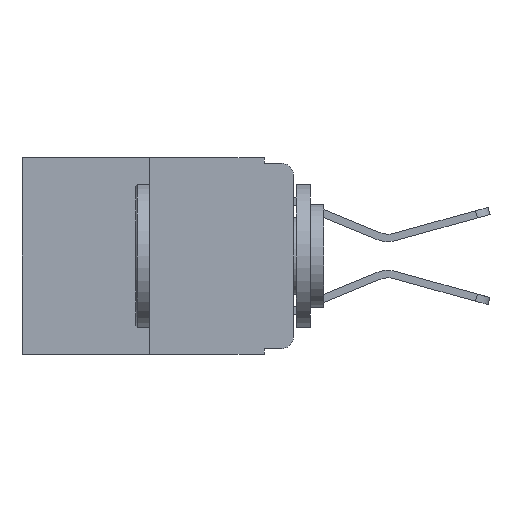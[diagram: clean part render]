
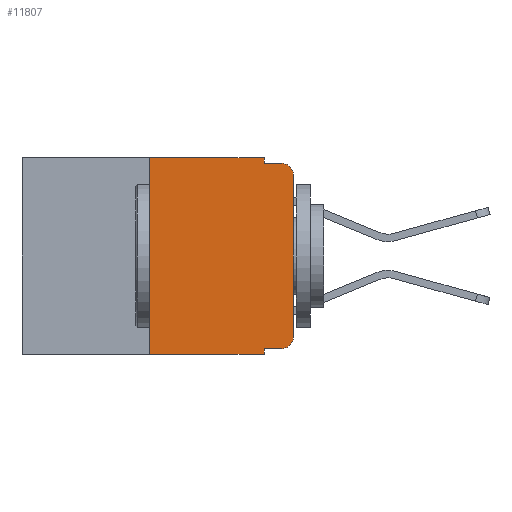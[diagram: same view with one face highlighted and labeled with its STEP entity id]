
A CAD part, left-side view. The second image highlights one B-rep face of the part: STEP entity #11807.
In plain terms, the highlighted planar face has unit normal (-1, 0, 0).
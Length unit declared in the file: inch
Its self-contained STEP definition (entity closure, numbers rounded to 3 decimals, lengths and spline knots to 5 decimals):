
#235 = ORIENTED_EDGE ( 'NONE', *, *, #6135, .F. ) ;
#460 = ORIENTED_EDGE ( 'NONE', *, *, #6069, .F. ) ;
#597 = LINE ( 'NONE', #14722, #12725 ) ;
#1324 = LINE ( 'NONE', #8059, #4423 ) ;
#1347 = DIRECTION ( 'NONE',  ( 0., 0., -1. ) ) ;
#1419 = VERTEX_POINT ( 'NONE', #8346 ) ;
#1439 = CARTESIAN_POINT ( 'NONE',  ( 0., 0.473, -0.343 ) ) ;
#1730 = LINE ( 'NONE', #14978, #10728 ) ;
#2251 = CARTESIAN_POINT ( 'NONE',  ( 0., 0.25, -0.343 ) ) ;
#2420 = CARTESIAN_POINT ( 'NONE',  ( 0., 0.051, -0.343 ) ) ;
#2587 = CARTESIAN_POINT ( 'NONE',  ( 0., 0.051, -0.01 ) ) ;
#2831 = DIRECTION ( 'NONE',  ( 0., -1., 0. ) ) ;
#3692 = ORIENTED_EDGE ( 'NONE', *, *, #5972, .T. ) ;
#3887 = ORIENTED_EDGE ( 'NONE', *, *, #6138, .T. ) ;
#3972 = CARTESIAN_POINT ( 'NONE',  ( 0., 0.25, 0. ) ) ;
#3984 = VECTOR ( 'NONE', #1347, 39.37008 ) ;
#4053 = VERTEX_POINT ( 'NONE', #5245 ) ;
#4377 = LINE ( 'NONE', #11861, #3984 ) ;
#4423 = VECTOR ( 'NONE', #5889, 39.37008 ) ;
#4670 = VERTEX_POINT ( 'NONE', #5679 ) ;
#5110 = DIRECTION ( 'NONE',  ( -1., 0., 0. ) ) ;
#5166 = EDGE_CURVE ( 'NONE', #1419, #8524, #1324, .T. ) ;
#5201 = PLANE ( 'NONE',  #5673 ) ;
#5245 = CARTESIAN_POINT ( 'NONE',  ( 0., 0.02, -0.333 ) ) ;
#5320 = CARTESIAN_POINT ( 'NONE',  ( 0., 0.051, -0.333 ) ) ;
#5601 = DIRECTION ( 'NONE',  ( -1., 0., 0. ) ) ;
#5673 = AXIS2_PLACEMENT_3D ( 'NONE', #13996, #7548, #15067 ) ;
#5679 = CARTESIAN_POINT ( 'NONE',  ( 0., 0.051, -0.333 ) ) ;
#5693 = EDGE_CURVE ( 'NONE', #7178, #12942, #8194, .T. ) ;
#5730 = CARTESIAN_POINT ( 'NONE',  ( 0., 0., -0.313 ) ) ;
#5889 = DIRECTION ( 'NONE',  ( 0., -1., 0. ) ) ;
#5972 = EDGE_CURVE ( 'NONE', #9551, #14573, #597, .T. ) ;
#6068 = EDGE_CURVE ( 'NONE', #14573, #13888, #11398, .T. ) ;
#6069 = EDGE_CURVE ( 'NONE', #8213, #13888, #13911, .T. ) ;
#6073 = CARTESIAN_POINT ( 'NONE',  ( 0., 0., -0.03 ) ) ;
#6095 = EDGE_CURVE ( 'NONE', #8524, #8213, #1730, .T. ) ;
#6115 = EDGE_CURVE ( 'NONE', #7178, #1419, #13583, .T. ) ;
#6135 = EDGE_CURVE ( 'NONE', #4670, #12942, #4377, .T. ) ;
#6138 = EDGE_CURVE ( 'NONE', #4670, #4053, #9695, .T. ) ;
#6201 = CARTESIAN_POINT ( 'NONE',  ( 0., 0.051, -0.01 ) ) ;
#6233 = EDGE_CURVE ( 'NONE', #4053, #9551, #8338, .T. ) ;
#6942 = ORIENTED_EDGE ( 'NONE', *, *, #6068, .T. ) ;
#7178 = VERTEX_POINT ( 'NONE', #2251 ) ;
#7277 = ORIENTED_EDGE ( 'NONE', *, *, #6095, .F. ) ;
#7548 = DIRECTION ( 'NONE',  ( 1., 0., 0. ) ) ;
#8059 = CARTESIAN_POINT ( 'NONE',  ( 0., 0.473, 0. ) ) ;
#8183 = VECTOR ( 'NONE', #9558, 39.37008 ) ;
#8194 = LINE ( 'NONE', #1439, #13591 ) ;
#8213 = VERTEX_POINT ( 'NONE', #6201 ) ;
#8246 = DIRECTION ( 'NONE',  ( 0., 0., 1. ) ) ;
#8338 = CIRCLE ( 'NONE', #11329, 0.02 ) ;
#8346 = CARTESIAN_POINT ( 'NONE',  ( 0., 0.25, 0. ) ) ;
#8516 = DIRECTION ( 'NONE',  ( 0., 0., -1. ) ) ;
#8524 = VERTEX_POINT ( 'NONE', #8769 ) ;
#8713 = FACE_OUTER_BOUND ( 'NONE', #12465, .T. ) ;
#8769 = CARTESIAN_POINT ( 'NONE',  ( 0., 0.051, 0. ) ) ;
#8912 = ORIENTED_EDGE ( 'NONE', *, *, #6115, .F. ) ;
#9551 = VERTEX_POINT ( 'NONE', #5730 ) ;
#9558 = DIRECTION ( 'NONE',  ( 0., -1., 0. ) ) ;
#9695 = LINE ( 'NONE', #5320, #12883 ) ;
#10383 = VECTOR ( 'NONE', #10756, 39.37008 ) ;
#10728 = VECTOR ( 'NONE', #8516, 39.37008 ) ;
#10756 = DIRECTION ( 'NONE',  ( 0., 0., 1. ) ) ;
#11329 = AXIS2_PLACEMENT_3D ( 'NONE', #12134, #5601, #13218 ) ;
#11398 = CIRCLE ( 'NONE', #14475, 0.02 ) ;
#11729 = CARTESIAN_POINT ( 'NONE',  ( 0., 0.02, -0.03 ) ) ;
#11807 = ADVANCED_FACE ( 'NONE', ( #8713 ), #5201, .F. ) ;
#11861 = CARTESIAN_POINT ( 'NONE',  ( 0., 0.051, 0. ) ) ;
#12134 = CARTESIAN_POINT ( 'NONE',  ( 0., 0.02, -0.313 ) ) ;
#12464 = ORIENTED_EDGE ( 'NONE', *, *, #5693, .T. ) ;
#12465 = EDGE_LOOP ( 'NONE', ( #3692, #6942, #460, #7277, #13651, #8912, #12464, #235, #3887, #12804 ) ) ;
#12698 = CARTESIAN_POINT ( 'NONE',  ( 0., 0.02, -0.01 ) ) ;
#12725 = VECTOR ( 'NONE', #8246, 39.37008 ) ;
#12804 = ORIENTED_EDGE ( 'NONE', *, *, #6233, .T. ) ;
#12806 = DIRECTION ( 'NONE',  ( 0., 0., -1. ) ) ;
#12883 = VECTOR ( 'NONE', #12984, 39.37008 ) ;
#12942 = VERTEX_POINT ( 'NONE', #2420 ) ;
#12984 = DIRECTION ( 'NONE',  ( 0., -1., 0. ) ) ;
#13218 = DIRECTION ( 'NONE',  ( 0., 0., -1. ) ) ;
#13583 = LINE ( 'NONE', #3972, #10383 ) ;
#13591 = VECTOR ( 'NONE', #2831, 39.37008 ) ;
#13651 = ORIENTED_EDGE ( 'NONE', *, *, #5166, .F. ) ;
#13888 = VERTEX_POINT ( 'NONE', #12698 ) ;
#13911 = LINE ( 'NONE', #2587, #8183 ) ;
#13996 = CARTESIAN_POINT ( 'NONE',  ( 0., 0.473, 0. ) ) ;
#14475 = AXIS2_PLACEMENT_3D ( 'NONE', #11729, #5110, #12806 ) ;
#14573 = VERTEX_POINT ( 'NONE', #6073 ) ;
#14722 = CARTESIAN_POINT ( 'NONE',  ( 0., 0., 0. ) ) ;
#14978 = CARTESIAN_POINT ( 'NONE',  ( 0., 0.051, 0. ) ) ;
#15067 = DIRECTION ( 'NONE',  ( 0., 0., -1. ) ) ;
